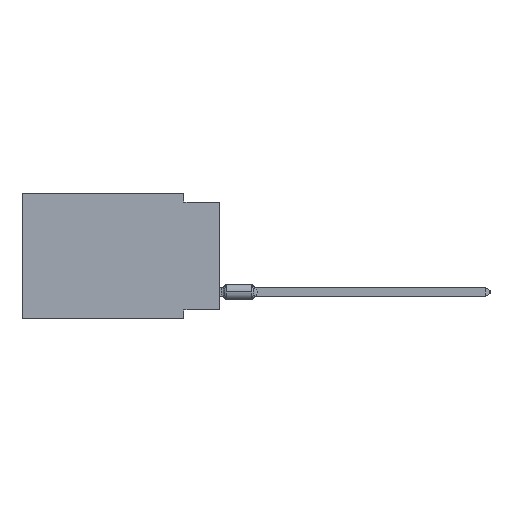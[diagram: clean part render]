
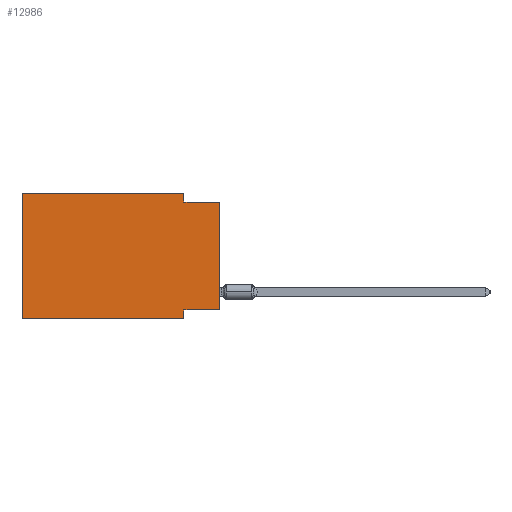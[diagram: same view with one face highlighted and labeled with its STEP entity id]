
A CAD part, left-side view. The second image highlights one B-rep face of the part: STEP entity #12986.
In plain terms, the highlighted planar face has unit normal (-1, 0, 0).
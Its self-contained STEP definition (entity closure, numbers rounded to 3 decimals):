
#366 = LINE ( 'NONE', #60644, #32073 ) ;
#553 = LINE ( 'NONE', #1255, #42503 ) ;
#1255 = CARTESIAN_POINT ( 'NONE',  ( 0., 13.97, 0. ) ) ;
#5923 = LINE ( 'NONE', #37489, #62418 ) ;
#7773 = ORIENTED_EDGE ( 'NONE', *, *, #22074, .T. ) ;
#8418 = EDGE_CURVE ( 'NONE', #20599, #36108, #5923, .T. ) ;
#8684 = DIRECTION ( 'NONE',  ( 1., 0., 0. ) ) ;
#11889 = DIRECTION ( 'NONE',  ( 0., -1., 0. ) ) ;
#12577 = FACE_OUTER_BOUND ( 'NONE', #67334, .T. ) ;
#12658 = DIRECTION ( 'NONE',  ( 0., 0., 1. ) ) ;
#12986 = ADVANCED_FACE ( 'NONE', ( #12577 ), #18528, .F. ) ;
#14101 = CARTESIAN_POINT ( 'NONE',  ( 0., 2.54, 0. ) ) ;
#14480 = CARTESIAN_POINT ( 'NONE',  ( 0., 2.54, -8.89 ) ) ;
#16592 = VECTOR ( 'NONE', #20655, 1000. ) ;
#17452 = ORIENTED_EDGE ( 'NONE', *, *, #30909, .F. ) ;
#18175 = CARTESIAN_POINT ( 'NONE',  ( 0., 0., -0.635 ) ) ;
#18528 = PLANE ( 'NONE',  #33627 ) ;
#19195 = VECTOR ( 'NONE', #65428, 1000. ) ;
#19269 = VERTEX_POINT ( 'NONE', #28082 ) ;
#19647 = CARTESIAN_POINT ( 'NONE',  ( 0., 0., -8.255 ) ) ;
#20599 = VERTEX_POINT ( 'NONE', #23622 ) ;
#20655 = DIRECTION ( 'NONE',  ( 0., 1., 0. ) ) ;
#22074 = EDGE_CURVE ( 'NONE', #65705, #47669, #366, .T. ) ;
#23146 = ORIENTED_EDGE ( 'NONE', *, *, #40665, .F. ) ;
#23622 = CARTESIAN_POINT ( 'NONE',  ( 0., 13.97, -8.89 ) ) ;
#25320 = ORIENTED_EDGE ( 'NONE', *, *, #45030, .F. ) ;
#27593 = LINE ( 'NONE', #50974, #19195 ) ;
#28082 = CARTESIAN_POINT ( 'NONE',  ( 0., 2.54, 0. ) ) ;
#30466 = CARTESIAN_POINT ( 'NONE',  ( 0., 2.54, -8.255 ) ) ;
#30909 = EDGE_CURVE ( 'NONE', #53634, #36108, #67737, .T. ) ;
#32073 = VECTOR ( 'NONE', #12658, 1000. ) ;
#33358 = VECTOR ( 'NONE', #45226, 1000. ) ;
#33627 = AXIS2_PLACEMENT_3D ( 'NONE', #40252, #8684, #45857 ) ;
#35419 = CARTESIAN_POINT ( 'NONE',  ( 0., 0., -8.255 ) ) ;
#35512 = DIRECTION ( 'NONE',  ( 0., 0., -1. ) ) ;
#36108 = VERTEX_POINT ( 'NONE', #61942 ) ;
#37489 = CARTESIAN_POINT ( 'NONE',  ( 0., 13.97, -8.89 ) ) ;
#40154 = CARTESIAN_POINT ( 'NONE',  ( 0., 2.54, -0.635 ) ) ;
#40252 = CARTESIAN_POINT ( 'NONE',  ( 0., 13.97, 0. ) ) ;
#40665 = EDGE_CURVE ( 'NONE', #20599, #46833, #44516, .T. ) ;
#40744 = DIRECTION ( 'NONE',  ( 0., 0., -1. ) ) ;
#41579 = EDGE_CURVE ( 'NONE', #19269, #45206, #51250, .T. ) ;
#42201 = VECTOR ( 'NONE', #40744, 1000. ) ;
#42503 = VECTOR ( 'NONE', #44044, 1000. ) ;
#44044 = DIRECTION ( 'NONE',  ( 0., -1., 0. ) ) ;
#44516 = LINE ( 'NONE', #65883, #33358 ) ;
#45030 = EDGE_CURVE ( 'NONE', #65705, #53634, #46957, .T. ) ;
#45206 = VERTEX_POINT ( 'NONE', #40154 ) ;
#45226 = DIRECTION ( 'NONE',  ( 0., 0., 1. ) ) ;
#45857 = DIRECTION ( 'NONE',  ( 0., 0., -1. ) ) ;
#46833 = VERTEX_POINT ( 'NONE', #60033 ) ;
#46957 = LINE ( 'NONE', #35419, #16592 ) ;
#47661 = ORIENTED_EDGE ( 'NONE', *, *, #52754, .F. ) ;
#47669 = VERTEX_POINT ( 'NONE', #18175 ) ;
#50974 = CARTESIAN_POINT ( 'NONE',  ( 0., 0., -0.635 ) ) ;
#51250 = LINE ( 'NONE', #14101, #42201 ) ;
#52754 = EDGE_CURVE ( 'NONE', #45206, #47669, #27593, .T. ) ;
#53634 = VERTEX_POINT ( 'NONE', #30466 ) ;
#55861 = VECTOR ( 'NONE', #35512, 1000. ) ;
#57711 = ORIENTED_EDGE ( 'NONE', *, *, #66395, .F. ) ;
#59114 = ORIENTED_EDGE ( 'NONE', *, *, #8418, .T. ) ;
#60033 = CARTESIAN_POINT ( 'NONE',  ( 0., 13.97, 0. ) ) ;
#60644 = CARTESIAN_POINT ( 'NONE',  ( 0., 0., 0. ) ) ;
#61942 = CARTESIAN_POINT ( 'NONE',  ( 0., 2.54, -8.89 ) ) ;
#62418 = VECTOR ( 'NONE', #11889, 1000. ) ;
#65428 = DIRECTION ( 'NONE',  ( 0., -1., 0. ) ) ;
#65705 = VERTEX_POINT ( 'NONE', #19647 ) ;
#65883 = CARTESIAN_POINT ( 'NONE',  ( 0., 13.97, 0. ) ) ;
#66395 = EDGE_CURVE ( 'NONE', #46833, #19269, #553, .T. ) ;
#67199 = ORIENTED_EDGE ( 'NONE', *, *, #41579, .F. ) ;
#67334 = EDGE_LOOP ( 'NONE', ( #7773, #47661, #67199, #57711, #23146, #59114, #17452, #25320 ) ) ;
#67737 = LINE ( 'NONE', #14480, #55861 ) ;
